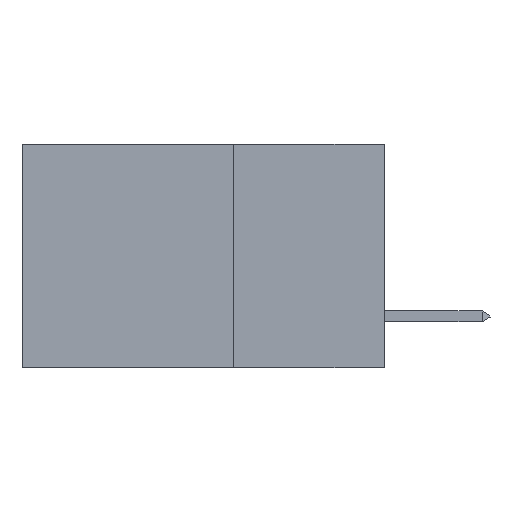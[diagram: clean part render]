
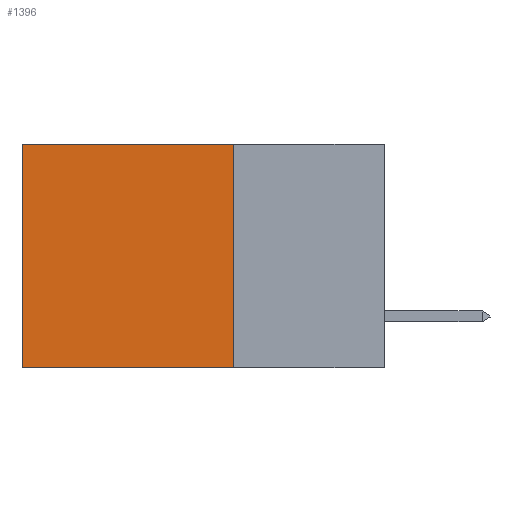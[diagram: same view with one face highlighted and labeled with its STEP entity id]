
A CAD part, left-side view. The second image highlights one B-rep face of the part: STEP entity #1396.
In plain terms, the highlighted planar face has unit normal (-1, 0, 0).
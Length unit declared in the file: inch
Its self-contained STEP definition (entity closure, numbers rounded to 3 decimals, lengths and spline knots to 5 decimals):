
#1289 = ORIENTED_EDGE ( 'NONE', *, *, #19682, .F. ) ;
#1380 = CARTESIAN_POINT ( 'NONE',  ( 0.2875, 0.25, 0. ) ) ;
#1396 = ADVANCED_FACE ( 'NONE', ( #9187 ), #21835, .F. ) ;
#1846 = VECTOR ( 'NONE', #9039, 39.37008 ) ;
#2134 = LINE ( 'NONE', #5269, #1846 ) ;
#4632 = CARTESIAN_POINT ( 'NONE',  ( 0.2875, 0.25, 0. ) ) ;
#4859 = LINE ( 'NONE', #1380, #14011 ) ;
#5269 = CARTESIAN_POINT ( 'NONE',  ( 0.2875, 0.25, -0.37 ) ) ;
#7050 = AXIS2_PLACEMENT_3D ( 'NONE', #9079, #7412, #16550 ) ;
#7412 = DIRECTION ( 'NONE',  ( 1., 0., 0. ) ) ;
#8149 = VERTEX_POINT ( 'NONE', #11197 ) ;
#8673 = DIRECTION ( 'NONE',  ( 0., 0., -1. ) ) ;
#9039 = DIRECTION ( 'NONE',  ( 0., 1., 0. ) ) ;
#9079 = CARTESIAN_POINT ( 'NONE',  ( 0.2875, 0.25, 0. ) ) ;
#9187 = FACE_OUTER_BOUND ( 'NONE', #13798, .T. ) ;
#9867 = VERTEX_POINT ( 'NONE', #19026 ) ;
#10197 = DIRECTION ( 'NONE',  ( 0., 0., -1. ) ) ;
#10569 = VECTOR ( 'NONE', #10197, 39.37008 ) ;
#11197 = CARTESIAN_POINT ( 'NONE',  ( 0.2875, 0.6, -0.37 ) ) ;
#11266 = EDGE_CURVE ( 'NONE', #14047, #9867, #4859, .T. ) ;
#11708 = CARTESIAN_POINT ( 'NONE',  ( 0.2875, 0.25, -0.37 ) ) ;
#11957 = CARTESIAN_POINT ( 'NONE',  ( 0.2875, 0.6, 0. ) ) ;
#12110 = DIRECTION ( 'NONE',  ( 0., 1., 0. ) ) ;
#13798 = EDGE_LOOP ( 'NONE', ( #16597, #1289, #18436, #23710 ) ) ;
#14011 = VECTOR ( 'NONE', #12110, 39.37008 ) ;
#14047 = VERTEX_POINT ( 'NONE', #4632 ) ;
#14116 = EDGE_CURVE ( 'NONE', #14047, #20263, #18139, .T. ) ;
#14992 = VECTOR ( 'NONE', #8673, 39.37008 ) ;
#16550 = DIRECTION ( 'NONE',  ( 0., 0., -1. ) ) ;
#16597 = ORIENTED_EDGE ( 'NONE', *, *, #23010, .T. ) ;
#17851 = CARTESIAN_POINT ( 'NONE',  ( 0.2875, 0.25, 0. ) ) ;
#18139 = LINE ( 'NONE', #17851, #14992 ) ;
#18258 = LINE ( 'NONE', #11957, #10569 ) ;
#18436 = ORIENTED_EDGE ( 'NONE', *, *, #14116, .F. ) ;
#19026 = CARTESIAN_POINT ( 'NONE',  ( 0.2875, 0.6, 0. ) ) ;
#19682 = EDGE_CURVE ( 'NONE', #20263, #8149, #2134, .T. ) ;
#20263 = VERTEX_POINT ( 'NONE', #11708 ) ;
#21835 = PLANE ( 'NONE',  #7050 ) ;
#23010 = EDGE_CURVE ( 'NONE', #9867, #8149, #18258, .T. ) ;
#23710 = ORIENTED_EDGE ( 'NONE', *, *, #11266, .T. ) ;
